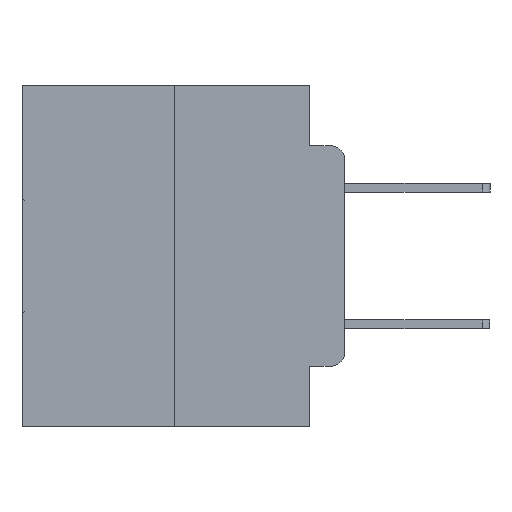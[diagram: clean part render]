
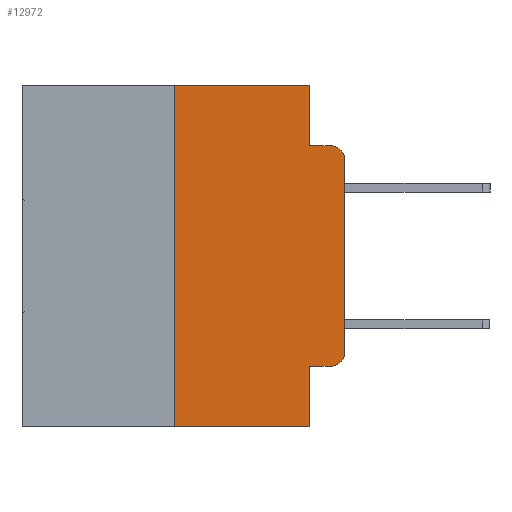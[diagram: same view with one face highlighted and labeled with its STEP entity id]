
A CAD part, left-side view. The second image highlights one B-rep face of the part: STEP entity #12972.
In plain terms, the highlighted planar face has unit normal (-1, 0, 0).
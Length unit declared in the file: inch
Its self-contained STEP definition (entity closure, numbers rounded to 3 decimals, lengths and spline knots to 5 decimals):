
#53 = VERTEX_POINT ( 'NONE', #71 ) ;
#59 = CARTESIAN_POINT ( 'NONE',  ( 0., 0.473, 0. ) ) ;
#71 = CARTESIAN_POINT ( 'NONE',  ( 0., 0.25, 0. ) ) ;
#654 = VERTEX_POINT ( 'NONE', #15367 ) ;
#737 = VERTEX_POINT ( 'NONE', #8255 ) ;
#1158 = EDGE_CURVE ( 'NONE', #53, #10975, #4486, .T. ) ;
#1174 = LINE ( 'NONE', #2099, #17787 ) ;
#1237 = DIRECTION ( 'NONE',  ( 0., 0., 1. ) ) ;
#1731 = VERTEX_POINT ( 'NONE', #23838 ) ;
#1858 = ORIENTED_EDGE ( 'NONE', *, *, #28827, .F. ) ;
#2092 = CARTESIAN_POINT ( 'NONE',  ( 0., 0.02, -0.4115 ) ) ;
#2099 = CARTESIAN_POINT ( 'NONE',  ( 0., 0.051, -0.0885 ) ) ;
#2413 = EDGE_CURVE ( 'NONE', #737, #654, #4775, .T. ) ;
#2752 = CIRCLE ( 'NONE', #24419, 0.02 ) ;
#2961 = DIRECTION ( 'NONE',  ( 0., 0., -1. ) ) ;
#3216 = CARTESIAN_POINT ( 'NONE',  ( 0., 0.051, -0.4115 ) ) ;
#3298 = VERTEX_POINT ( 'NONE', #2092 ) ;
#3393 = CARTESIAN_POINT ( 'NONE',  ( 0., 0.051, -0.4115 ) ) ;
#4394 = ORIENTED_EDGE ( 'NONE', *, *, #21045, .F. ) ;
#4471 = VECTOR ( 'NONE', #21379, 39.37008 ) ;
#4486 = LINE ( 'NONE', #59, #27662 ) ;
#4775 = LINE ( 'NONE', #22123, #10686 ) ;
#5075 = ORIENTED_EDGE ( 'NONE', *, *, #18351, .T. ) ;
#5124 = LINE ( 'NONE', #26516, #18483 ) ;
#6101 = VERTEX_POINT ( 'NONE', #3216 ) ;
#6468 = ORIENTED_EDGE ( 'NONE', *, *, #19865, .F. ) ;
#6671 = EDGE_CURVE ( 'NONE', #6101, #3298, #10416, .T. ) ;
#6958 = VECTOR ( 'NONE', #21828, 39.37008 ) ;
#7379 = CARTESIAN_POINT ( 'NONE',  ( 0., 0.473, 0. ) ) ;
#7390 = VECTOR ( 'NONE', #1237, 39.37008 ) ;
#8086 = LINE ( 'NONE', #17042, #7390 ) ;
#8255 = CARTESIAN_POINT ( 'NONE',  ( 0., 0.25, -0.5 ) ) ;
#8292 = DIRECTION ( 'NONE',  ( 0., 0., -1. ) ) ;
#10287 = CARTESIAN_POINT ( 'NONE',  ( 0., 0.051, -0.0885 ) ) ;
#10304 = DIRECTION ( 'NONE',  ( 0., -1., 0. ) ) ;
#10416 = LINE ( 'NONE', #3393, #4471 ) ;
#10601 = DIRECTION ( 'NONE',  ( 0., -1., 0. ) ) ;
#10686 = VECTOR ( 'NONE', #10304, 39.37008 ) ;
#10975 = VERTEX_POINT ( 'NONE', #11925 ) ;
#11696 = CARTESIAN_POINT ( 'NONE',  ( 0., 0.02, -0.1085 ) ) ;
#11925 = CARTESIAN_POINT ( 'NONE',  ( 0., 0.051, 0. ) ) ;
#12061 = ORIENTED_EDGE ( 'NONE', *, *, #13206, .F. ) ;
#12163 = AXIS2_PLACEMENT_3D ( 'NONE', #7379, #16421, #2961 ) ;
#12261 = EDGE_CURVE ( 'NONE', #24099, #22231, #2752, .T. ) ;
#12296 = CARTESIAN_POINT ( 'NONE',  ( 0., 0.02, -0.3915 ) ) ;
#12972 = ADVANCED_FACE ( 'NONE', ( #19288 ), #14112, .F. ) ;
#13012 = DIRECTION ( 'NONE',  ( 0., 0., -1. ) ) ;
#13113 = ORIENTED_EDGE ( 'NONE', *, *, #23479, .T. ) ;
#13206 = EDGE_CURVE ( 'NONE', #737, #53, #18932, .T. ) ;
#13954 = DIRECTION ( 'NONE',  ( 0., 0., -1. ) ) ;
#14112 = PLANE ( 'NONE',  #12163 ) ;
#14574 = DIRECTION ( 'NONE',  ( 0., 0., -1. ) ) ;
#14974 = VERTEX_POINT ( 'NONE', #10287 ) ;
#15043 = CARTESIAN_POINT ( 'NONE',  ( 0., 0.051, 0. ) ) ;
#15367 = CARTESIAN_POINT ( 'NONE',  ( 0., 0.051, -0.5 ) ) ;
#16329 = ORIENTED_EDGE ( 'NONE', *, *, #6671, .T. ) ;
#16421 = DIRECTION ( 'NONE',  ( 1., 0., 0. ) ) ;
#17042 = CARTESIAN_POINT ( 'NONE',  ( 0., 0., 0. ) ) ;
#17715 = ORIENTED_EDGE ( 'NONE', *, *, #12261, .T. ) ;
#17787 = VECTOR ( 'NONE', #20131, 39.37008 ) ;
#18144 = CARTESIAN_POINT ( 'NONE',  ( 0., 0., -0.1085 ) ) ;
#18351 = EDGE_CURVE ( 'NONE', #1731, #24099, #8086, .T. ) ;
#18483 = VECTOR ( 'NONE', #13012, 39.37008 ) ;
#18932 = LINE ( 'NONE', #19560, #6958 ) ;
#19213 = CARTESIAN_POINT ( 'NONE',  ( 0., 0.02, -0.0885 ) ) ;
#19288 = FACE_OUTER_BOUND ( 'NONE', #19989, .T. ) ;
#19560 = CARTESIAN_POINT ( 'NONE',  ( 0., 0.25, 0. ) ) ;
#19845 = ORIENTED_EDGE ( 'NONE', *, *, #1158, .F. ) ;
#19865 = EDGE_CURVE ( 'NONE', #14974, #22231, #1174, .T. ) ;
#19989 = EDGE_LOOP ( 'NONE', ( #5075, #17715, #6468, #1858, #19845, #12061, #20214, #4394, #16329, #13113 ) ) ;
#20131 = DIRECTION ( 'NONE',  ( 0., -1., 0. ) ) ;
#20214 = ORIENTED_EDGE ( 'NONE', *, *, #2413, .T. ) ;
#21045 = EDGE_CURVE ( 'NONE', #6101, #654, #5124, .T. ) ;
#21379 = DIRECTION ( 'NONE',  ( 0., -1., 0. ) ) ;
#21828 = DIRECTION ( 'NONE',  ( 0., 0., 1. ) ) ;
#22123 = CARTESIAN_POINT ( 'NONE',  ( 0., 0.473, -0.5 ) ) ;
#22231 = VERTEX_POINT ( 'NONE', #19213 ) ;
#23479 = EDGE_CURVE ( 'NONE', #3298, #1731, #27082, .T. ) ;
#23838 = CARTESIAN_POINT ( 'NONE',  ( 0., 0., -0.3915 ) ) ;
#24099 = VERTEX_POINT ( 'NONE', #18144 ) ;
#24419 = AXIS2_PLACEMENT_3D ( 'NONE', #11696, #27435, #13954 ) ;
#25368 = AXIS2_PLACEMENT_3D ( 'NONE', #12296, #28047, #14574 ) ;
#26232 = VECTOR ( 'NONE', #8292, 39.37008 ) ;
#26516 = CARTESIAN_POINT ( 'NONE',  ( 0., 0.051, 0. ) ) ;
#26927 = LINE ( 'NONE', #15043, #26232 ) ;
#27082 = CIRCLE ( 'NONE', #25368, 0.02 ) ;
#27435 = DIRECTION ( 'NONE',  ( -1., 0., 0. ) ) ;
#27662 = VECTOR ( 'NONE', #10601, 39.37008 ) ;
#28047 = DIRECTION ( 'NONE',  ( -1., 0., 0. ) ) ;
#28827 = EDGE_CURVE ( 'NONE', #10975, #14974, #26927, .T. ) ;
